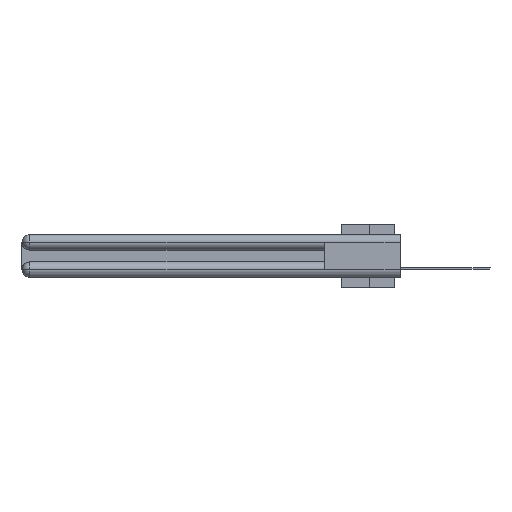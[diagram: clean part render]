
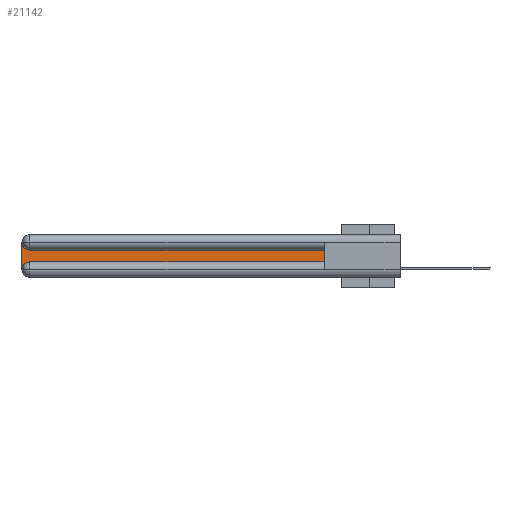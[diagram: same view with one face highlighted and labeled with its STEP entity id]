
A CAD part, left-side view. The second image highlights one B-rep face of the part: STEP entity #21142.
In plain terms, the highlighted planar face has unit normal (-1, 0, 0).
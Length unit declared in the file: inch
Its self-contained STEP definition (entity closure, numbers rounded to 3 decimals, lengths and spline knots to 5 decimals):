
#423 = EDGE_CURVE ( 'NONE', #25187, #9852, #10852, .T. ) ;
#549 = LINE ( 'NONE', #37468, #16042 ) ;
#1908 = EDGE_CURVE ( 'NONE', #3588, #25187, #26197, .T. ) ;
#2146 = EDGE_CURVE ( 'NONE', #32188, #3588, #7287, .T. ) ;
#2172 = DIRECTION ( 'NONE',  ( 0., 0., -1. ) ) ;
#2596 = EDGE_CURVE ( 'NONE', #13366, #34890, #549, .T. ) ;
#3588 = VERTEX_POINT ( 'NONE', #27200 ) ;
#3717 = CARTESIAN_POINT ( 'NONE',  ( 0.075, 2.94, -0.0625 ) ) ;
#3862 = DIRECTION ( 'NONE',  ( 1., 0., 0. ) ) ;
#4595 = VECTOR ( 'NONE', #20231, 39.37008 ) ;
#4912 = EDGE_CURVE ( 'NONE', #9852, #13366, #25053, .T. ) ;
#5167 = ORIENTED_EDGE ( 'NONE', *, *, #13859, .T. ) ;
#7287 = LINE ( 'NONE', #28874, #31958 ) ;
#9852 = VERTEX_POINT ( 'NONE', #38051 ) ;
#10017 = CIRCLE ( 'NONE', #31778, 0.06 ) ;
#10539 = FACE_OUTER_BOUND ( 'NONE', #37983, .T. ) ;
#10852 = LINE ( 'NONE', #38186, #4595 ) ;
#13366 = VERTEX_POINT ( 'NONE', #25676 ) ;
#13577 = AXIS2_PLACEMENT_3D ( 'NONE', #16915, #26245, #2172 ) ;
#13859 = EDGE_CURVE ( 'NONE', #34890, #32188, #10017, .T. ) ;
#15885 = DIRECTION ( 'NONE',  ( 0., 1., 0. ) ) ;
#16034 = DIRECTION ( 'NONE',  ( 0., 0., -1. ) ) ;
#16042 = VECTOR ( 'NONE', #15885, 39.37008 ) ;
#16564 = ORIENTED_EDGE ( 'NONE', *, *, #1908, .T. ) ;
#16730 = CARTESIAN_POINT ( 'NONE',  ( 0.075, 3., -0.0625 ) ) ;
#16915 = CARTESIAN_POINT ( 'NONE',  ( 0.075, 3., -0.1225 ) ) ;
#20231 = DIRECTION ( 'NONE',  ( 0., -1., 0. ) ) ;
#21142 = ADVANCED_FACE ( 'NONE', ( #10539 ), #32326, .F. ) ;
#21832 = DIRECTION ( 'NONE',  ( 0., 0., 1. ) ) ;
#23118 = VECTOR ( 'NONE', #21832, 39.37008 ) ;
#24314 = CARTESIAN_POINT ( 'NONE',  ( 0.075, 2.94, -0.1225 ) ) ;
#24986 = DIRECTION ( 'NONE',  ( 0., 0., -1. ) ) ;
#25053 = LINE ( 'NONE', #31005, #23118 ) ;
#25187 = VERTEX_POINT ( 'NONE', #27758 ) ;
#25517 = CARTESIAN_POINT ( 'NONE',  ( 0.075, 2.94, -0.2775 ) ) ;
#25676 = CARTESIAN_POINT ( 'NONE',  ( 0.075, 0.6, -0.1225 ) ) ;
#26197 = CIRCLE ( 'NONE', #33519, 0.06 ) ;
#26245 = DIRECTION ( 'NONE',  ( 1., 0., 0. ) ) ;
#27200 = CARTESIAN_POINT ( 'NONE',  ( 0.075, 3., -0.2775 ) ) ;
#27758 = CARTESIAN_POINT ( 'NONE',  ( 0.075, 2.94, -0.2175 ) ) ;
#28874 = CARTESIAN_POINT ( 'NONE',  ( 0.075, 3., -0.2175 ) ) ;
#31005 = CARTESIAN_POINT ( 'NONE',  ( 0.075, 0.6, -0.2175 ) ) ;
#31778 = AXIS2_PLACEMENT_3D ( 'NONE', #3717, #3862, #16034 ) ;
#31958 = VECTOR ( 'NONE', #32112, 39.37008 ) ;
#32112 = DIRECTION ( 'NONE',  ( 0., 0., -1. ) ) ;
#32188 = VERTEX_POINT ( 'NONE', #16730 ) ;
#32326 = PLANE ( 'NONE',  #13577 ) ;
#33519 = AXIS2_PLACEMENT_3D ( 'NONE', #25517, #37516, #24986 ) ;
#34305 = ORIENTED_EDGE ( 'NONE', *, *, #423, .T. ) ;
#34890 = VERTEX_POINT ( 'NONE', #24314 ) ;
#37468 = CARTESIAN_POINT ( 'NONE',  ( 0.075, 0.6, -0.1225 ) ) ;
#37516 = DIRECTION ( 'NONE',  ( 1., 0., 0. ) ) ;
#37983 = EDGE_LOOP ( 'NONE', ( #37987, #5167, #39462, #16564, #34305, #39628 ) ) ;
#37987 = ORIENTED_EDGE ( 'NONE', *, *, #2596, .T. ) ;
#38051 = CARTESIAN_POINT ( 'NONE',  ( 0.075, 0.6, -0.2175 ) ) ;
#38186 = CARTESIAN_POINT ( 'NONE',  ( 0.075, 0.6, -0.2175 ) ) ;
#39462 = ORIENTED_EDGE ( 'NONE', *, *, #2146, .T. ) ;
#39628 = ORIENTED_EDGE ( 'NONE', *, *, #4912, .T. ) ;
